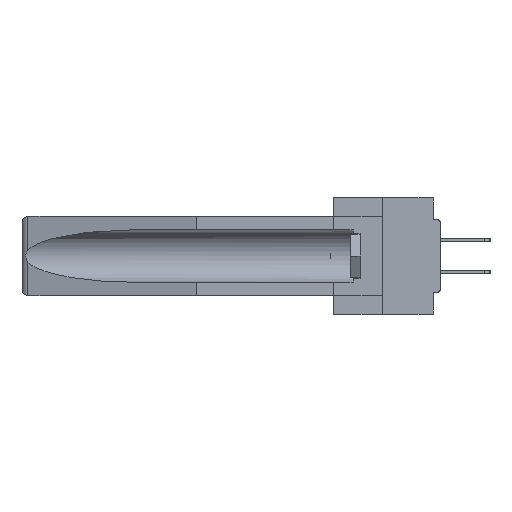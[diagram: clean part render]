
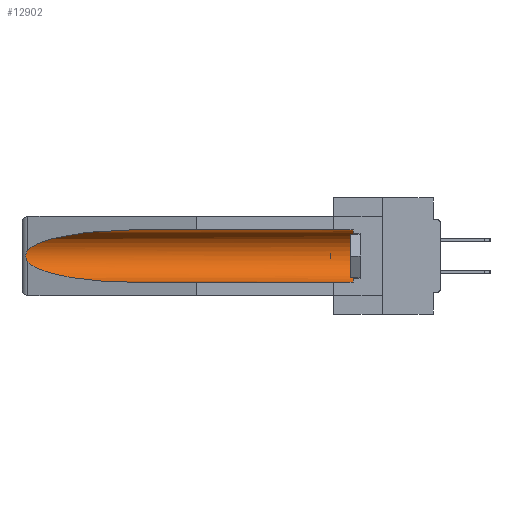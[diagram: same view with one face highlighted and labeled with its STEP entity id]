
A CAD part, left-side view. The second image highlights one B-rep face of the part: STEP entity #12902.
In plain terms, the highlighted cylindrical face has radius 2.857 mm (diameter 5.715 mm), a partial arc.
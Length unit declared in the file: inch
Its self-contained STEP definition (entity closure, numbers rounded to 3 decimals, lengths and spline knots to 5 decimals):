
#2186 = CARTESIAN_POINT ( 'NONE',  ( 0.26537, 1.52718, -0.14972 ) ) ;
#2431 = CARTESIAN_POINT ( 'NONE',  ( 0.2675, 1.53308, -0.16763 ) ) ;
#2790 = CARTESIAN_POINT ( 'NONE',  ( 0.155, 0.126, -0.284 ) ) ;
#2863 =( BOUNDED_CURVE ( )  B_SPLINE_CURVE ( 3, ( #39679, #17176, #6326, #6163 ),
 .UNSPECIFIED., .F., .T. ) 
 B_SPLINE_CURVE_WITH_KNOTS ( ( 4, 4 ),
 ( 0.1948, 1.5708 ),
 .UNSPECIFIED. ) 
 CURVE ( )  GEOMETRIC_REPRESENTATION_ITEM ( )  RATIONAL_B_SPLINE_CURVE ( ( 1., 0.848, 0.848, 1. ) ) 
 REPRESENTATION_ITEM ( '' )  );
#4951 = CARTESIAN_POINT ( 'NONE',  ( 0.155, 1.07973, -0.284 ) ) ;
#5945 = VERTEX_POINT ( 'NONE', #4951 ) ;
#6163 = CARTESIAN_POINT ( 'NONE',  ( 0.155, 1.07973, -0.284 ) ) ;
#6326 = CARTESIAN_POINT ( 'NONE',  ( 0.21114, 1.30732, -0.284 ) ) ;
#7808 = DIRECTION ( 'NONE',  ( 0., -1., 0. ) ) ;
#9722 = CARTESIAN_POINT ( 'NONE',  ( 0.26654, 1.53092, -0.15636 ) ) ;
#9795 = CARTESIAN_POINT ( 'NONE',  ( 0.25451, 1.48313, -0.09465 ) ) ;
#10550 = EDGE_CURVE ( 'NONE', #25629, #5945, #44803, .T. ) ;
#11527 = DIRECTION ( 'NONE',  ( 0., 1., 0. ) ) ;
#12333 = VERTEX_POINT ( 'NONE', #42710 ) ;
#12507 = VERTEX_POINT ( 'NONE', #33117 ) ;
#12902 = ADVANCED_FACE ( 'NONE', ( #48732 ), #13416, .F. ) ;
#13416 = CYLINDRICAL_SURFACE ( 'NONE', #31793, 0.1125 ) ;
#14235 = VECTOR ( 'NONE', #33510, 39.37008 ) ;
#14405 = EDGE_CURVE ( 'NONE', #31059, #25598, #32131, .T. ) ;
#16805 = CARTESIAN_POINT ( 'NONE',  ( 0.26537, 1.52718, -0.19328 ) ) ;
#16942 = ORIENTED_EDGE ( 'NONE', *, *, #46904, .T. ) ;
#17108 = CARTESIAN_POINT ( 'NONE',  ( 0.2675, 1.53308, -0.17534 ) ) ;
#17176 = CARTESIAN_POINT ( 'NONE',  ( 0.25451, 1.48313, -0.24835 ) ) ;
#18877 =( BOUNDED_CURVE ( )  B_SPLINE_CURVE ( 3, ( #28840, #20791, #9795, #2186 ),
 .UNSPECIFIED., .F., .F. ) 
 B_SPLINE_CURVE_WITH_KNOTS ( ( 4, 4 ),
 ( 4.71239, 6.08839 ),
 .UNSPECIFIED. ) 
 CURVE ( )  GEOMETRIC_REPRESENTATION_ITEM ( )  RATIONAL_B_SPLINE_CURVE ( ( 1., 0.848, 0.848, 1. ) ) 
 REPRESENTATION_ITEM ( '' )  );
#19168 = DIRECTION ( 'NONE',  ( 0., 0., 1. ) ) ;
#20769 = CARTESIAN_POINT ( 'NONE',  ( 0.155, -0.30754, -0.1715 ) ) ;
#20791 = CARTESIAN_POINT ( 'NONE',  ( 0.21114, 1.30732, -0.059 ) ) ;
#22216 = AXIS2_PLACEMENT_3D ( 'NONE', #38224, #7808, #19168 ) ;
#22422 = ORIENTED_EDGE ( 'NONE', *, *, #10550, .F. ) ;
#24842 = CARTESIAN_POINT ( 'NONE',  ( 0.26537, 1.52718, -0.19328 ) ) ;
#25598 = VERTEX_POINT ( 'NONE', #16805 ) ;
#25629 = VERTEX_POINT ( 'NONE', #2790 ) ;
#25838 = LINE ( 'NONE', #26501, #32883 ) ;
#25857 = EDGE_CURVE ( 'NONE', #12333, #12507, #25838, .T. ) ;
#26501 = CARTESIAN_POINT ( 'NONE',  ( 0.155, -0.30754, -0.059 ) ) ;
#28049 = DIRECTION ( 'NONE',  ( 0., 0., 1. ) ) ;
#28455 = CARTESIAN_POINT ( 'NONE',  ( 0.26537, 1.52718, -0.14972 ) ) ;
#28840 = CARTESIAN_POINT ( 'NONE',  ( 0.155, 1.07973, -0.059 ) ) ;
#31059 = VERTEX_POINT ( 'NONE', #33628 ) ;
#31530 = EDGE_CURVE ( 'NONE', #12507, #31059, #18877, .T. ) ;
#31793 = AXIS2_PLACEMENT_3D ( 'NONE', #20769, #46601, #28049 ) ;
#31912 = CARTESIAN_POINT ( 'NONE',  ( 0.2673, 1.5327, -0.16383 ) ) ;
#31947 = ORIENTED_EDGE ( 'NONE', *, *, #31530, .T. ) ;
#32131 = B_SPLINE_CURVE_WITH_KNOTS ( 'NONE', 3,
 ( #28455, #32228, #9722, #31912, #2431, #17108, #39924, #35689, #43711, #24842 ),
 .UNSPECIFIED., .F., .F.,
 ( 4, 2, 2, 2, 4 ),
 ( 0., 0.00029, 0.00058, 0.00087, 0.00117 ),
 .UNSPECIFIED. ) ;
#32228 = CARTESIAN_POINT ( 'NONE',  ( 0.26597, 1.52961, -0.15275 ) ) ;
#32883 = VECTOR ( 'NONE', #11527, 39.37008 ) ;
#33117 = CARTESIAN_POINT ( 'NONE',  ( 0.155, 1.07973, -0.059 ) ) ;
#33510 = DIRECTION ( 'NONE',  ( 0., 1., 0. ) ) ;
#33557 = EDGE_CURVE ( 'NONE', #25629, #12333, #45301, .T. ) ;
#33628 = CARTESIAN_POINT ( 'NONE',  ( 0.26537, 1.52718, -0.14972 ) ) ;
#34543 = ORIENTED_EDGE ( 'NONE', *, *, #33557, .T. ) ;
#35523 = EDGE_LOOP ( 'NONE', ( #31947, #47271, #16942, #22422, #34543, #42183 ) ) ;
#35689 = CARTESIAN_POINT ( 'NONE',  ( 0.26655, 1.53094, -0.18657 ) ) ;
#36948 = CARTESIAN_POINT ( 'NONE',  ( 0.155, -0.30754, -0.284 ) ) ;
#38224 = CARTESIAN_POINT ( 'NONE',  ( 0.155, 0.126, -0.1715 ) ) ;
#39679 = CARTESIAN_POINT ( 'NONE',  ( 0.26537, 1.52718, -0.19328 ) ) ;
#39924 = CARTESIAN_POINT ( 'NONE',  ( 0.2673, 1.53269, -0.17917 ) ) ;
#42183 = ORIENTED_EDGE ( 'NONE', *, *, #25857, .T. ) ;
#42710 = CARTESIAN_POINT ( 'NONE',  ( 0.155, 0.126, -0.059 ) ) ;
#43711 = CARTESIAN_POINT ( 'NONE',  ( 0.26597, 1.5296, -0.19026 ) ) ;
#44803 = LINE ( 'NONE', #36948, #14235 ) ;
#45301 = CIRCLE ( 'NONE', #22216, 0.1125 ) ;
#46601 = DIRECTION ( 'NONE',  ( 0., 1., 0. ) ) ;
#46904 = EDGE_CURVE ( 'NONE', #25598, #5945, #2863, .T. ) ;
#47271 = ORIENTED_EDGE ( 'NONE', *, *, #14405, .T. ) ;
#48732 = FACE_OUTER_BOUND ( 'NONE', #35523, .T. ) ;
